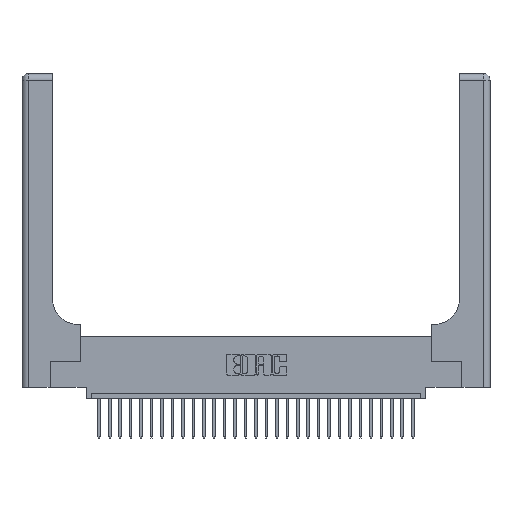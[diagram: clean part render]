
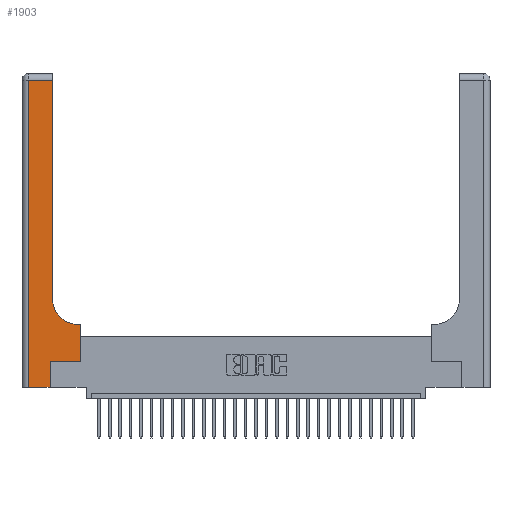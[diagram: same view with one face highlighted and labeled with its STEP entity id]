
A CAD part, top view. The second image highlights one B-rep face of the part: STEP entity #1903.
In plain terms, the highlighted planar face has unit normal (0, 0, 1).
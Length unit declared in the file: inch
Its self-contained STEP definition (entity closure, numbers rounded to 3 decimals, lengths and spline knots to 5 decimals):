
#2 = LINE ( 'NONE', #16142, #11692 ) ;
#324 = PLANE ( 'NONE',  #11605 ) ;
#544 = ORIENTED_EDGE ( 'NONE', *, *, #15474, .T. ) ;
#896 = EDGE_CURVE ( 'NONE', #22609, #7328, #19361, .T. ) ;
#1109 = CARTESIAN_POINT ( 'NONE',  ( 0.5585, 0.25, 0.37 ) ) ;
#1841 = CARTESIAN_POINT ( 'NONE',  ( 0.2915, 0.85, 0.37 ) ) ;
#1903 = ADVANCED_FACE ( 'NONE', ( #6975 ), #324, .F. ) ;
#2253 = DIRECTION ( 'NONE',  ( 1., 0., 0. ) ) ;
#2423 = DIRECTION ( 'NONE',  ( 0., 1., 0. ) ) ;
#2860 = CARTESIAN_POINT ( 'NONE',  ( 0.269, 0.25, 0.37 ) ) ;
#3517 = ORIENTED_EDGE ( 'NONE', *, *, #15906, .T. ) ;
#4789 = CARTESIAN_POINT ( 'NONE',  ( 0.5585, 0.6, 0.37 ) ) ;
#4871 = CARTESIAN_POINT ( 'NONE',  ( 0.269, 0., 0.37 ) ) ;
#4964 = DIRECTION ( 'NONE',  ( 1., 0., 0. ) ) ;
#5038 = LINE ( 'NONE', #6964, #18498 ) ;
#5293 = CARTESIAN_POINT ( 'NONE',  ( 0.269, 0., 0.37 ) ) ;
#5544 = DIRECTION ( 'NONE',  ( 0., 0., -1. ) ) ;
#6826 = LINE ( 'NONE', #15945, #17736 ) ;
#6964 = CARTESIAN_POINT ( 'NONE',  ( 0., 0., 0.37 ) ) ;
#6975 = FACE_OUTER_BOUND ( 'NONE', #15168, .T. ) ;
#7288 = VERTEX_POINT ( 'NONE', #13985 ) ;
#7328 = VERTEX_POINT ( 'NONE', #1841 ) ;
#7379 = ORIENTED_EDGE ( 'NONE', *, *, #8226, .T. ) ;
#7562 = VECTOR ( 'NONE', #2423, 39.37008 ) ;
#7746 = ORIENTED_EDGE ( 'NONE', *, *, #17480, .T. ) ;
#8226 = EDGE_CURVE ( 'NONE', #7328, #9029, #23902, .T. ) ;
#8931 = EDGE_CURVE ( 'NONE', #26840, #21316, #24236, .T. ) ;
#9029 = VERTEX_POINT ( 'NONE', #24638 ) ;
#9257 = CARTESIAN_POINT ( 'NONE',  ( 0.5415, 0.6, 0.37 ) ) ;
#9568 = CARTESIAN_POINT ( 'NONE',  ( 0.269, 0.25, 0.37 ) ) ;
#9835 = VERTEX_POINT ( 'NONE', #20482 ) ;
#9951 = DIRECTION ( 'NONE',  ( -1., 0., 0. ) ) ;
#10980 = LINE ( 'NONE', #19491, #13154 ) ;
#11176 = EDGE_CURVE ( 'NONE', #21316, #22609, #10980, .T. ) ;
#11213 = ORIENTED_EDGE ( 'NONE', *, *, #11176, .T. ) ;
#11605 = AXIS2_PLACEMENT_3D ( 'NONE', #17251, #5544, #9951 ) ;
#11692 = VECTOR ( 'NONE', #20890, 39.37008 ) ;
#11893 = VECTOR ( 'NONE', #26835, 39.37008 ) ;
#12003 = EDGE_CURVE ( 'NONE', #7288, #29680, #5038, .T. ) ;
#12397 = ORIENTED_EDGE ( 'NONE', *, *, #12003, .T. ) ;
#13154 = VECTOR ( 'NONE', #19591, 39.37008 ) ;
#13660 = VERTEX_POINT ( 'NONE', #2860 ) ;
#13985 = CARTESIAN_POINT ( 'NONE',  ( 0.06, 0., 0.37 ) ) ;
#15168 = EDGE_LOOP ( 'NONE', ( #7379, #23730, #7746, #12397, #3517, #544, #22151, #11213, #15201 ) ) ;
#15201 = ORIENTED_EDGE ( 'NONE', *, *, #896, .T. ) ;
#15394 = CARTESIAN_POINT ( 'NONE',  ( 0.5585, 0.25, 0.37 ) ) ;
#15474 = EDGE_CURVE ( 'NONE', #13660, #26840, #21424, .T. ) ;
#15906 = EDGE_CURVE ( 'NONE', #29680, #13660, #17481, .T. ) ;
#15945 = CARTESIAN_POINT ( 'NONE',  ( 0.06, 3., 0.37 ) ) ;
#16106 = CARTESIAN_POINT ( 'NONE',  ( 0.5415, 0.85, 0.37 ) ) ;
#16142 = CARTESIAN_POINT ( 'NONE',  ( 0., 2.94, 0.37 ) ) ;
#17251 = CARTESIAN_POINT ( 'NONE',  ( 0., 3., 0.37 ) ) ;
#17421 = AXIS2_PLACEMENT_3D ( 'NONE', #16106, #23189, #2253 ) ;
#17480 = EDGE_CURVE ( 'NONE', #9835, #7288, #6826, .T. ) ;
#17481 = LINE ( 'NONE', #4871, #22925 ) ;
#17736 = VECTOR ( 'NONE', #27534, 39.37008 ) ;
#18498 = VECTOR ( 'NONE', #27978, 39.37008 ) ;
#18613 = CARTESIAN_POINT ( 'NONE',  ( 0.2915, 3., 0.37 ) ) ;
#19361 = CIRCLE ( 'NONE', #17421, 0.25 ) ;
#19491 = CARTESIAN_POINT ( 'NONE',  ( 0.2915, 0.6, 0.37 ) ) ;
#19591 = DIRECTION ( 'NONE',  ( -1., 0., 0. ) ) ;
#19988 = VECTOR ( 'NONE', #4964, 39.37008 ) ;
#20482 = CARTESIAN_POINT ( 'NONE',  ( 0.06, 2.94, 0.37 ) ) ;
#20890 = DIRECTION ( 'NONE',  ( -1., 0., 0. ) ) ;
#21316 = VERTEX_POINT ( 'NONE', #4789 ) ;
#21424 = LINE ( 'NONE', #9568, #19988 ) ;
#22151 = ORIENTED_EDGE ( 'NONE', *, *, #8931, .T. ) ;
#22377 = DIRECTION ( 'NONE',  ( 0., 1., 0. ) ) ;
#22609 = VERTEX_POINT ( 'NONE', #9257 ) ;
#22925 = VECTOR ( 'NONE', #22377, 39.37008 ) ;
#23189 = DIRECTION ( 'NONE',  ( 0., 0., -1. ) ) ;
#23730 = ORIENTED_EDGE ( 'NONE', *, *, #25841, .T. ) ;
#23902 = LINE ( 'NONE', #18613, #7562 ) ;
#24236 = LINE ( 'NONE', #1109, #11893 ) ;
#24638 = CARTESIAN_POINT ( 'NONE',  ( 0.2915, 2.94, 0.37 ) ) ;
#25841 = EDGE_CURVE ( 'NONE', #9029, #9835, #2, .T. ) ;
#26835 = DIRECTION ( 'NONE',  ( 0., 1., 0. ) ) ;
#26840 = VERTEX_POINT ( 'NONE', #15394 ) ;
#27534 = DIRECTION ( 'NONE',  ( 0., -1., 0. ) ) ;
#27978 = DIRECTION ( 'NONE',  ( 1., 0., 0. ) ) ;
#29680 = VERTEX_POINT ( 'NONE', #5293 ) ;
